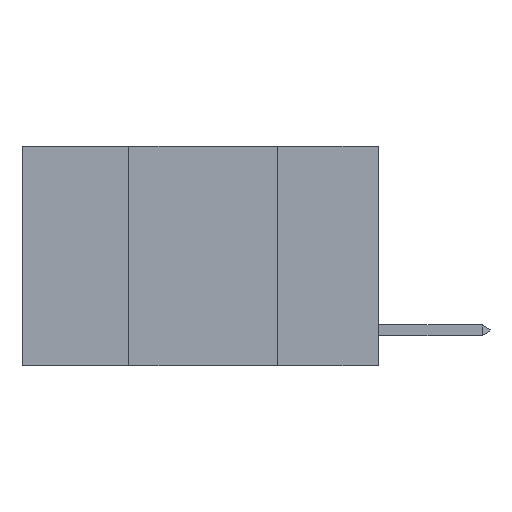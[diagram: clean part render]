
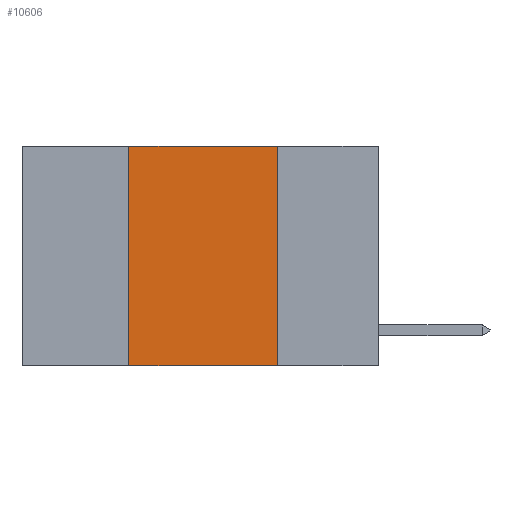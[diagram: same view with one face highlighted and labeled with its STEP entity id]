
A CAD part, left-side view. The second image highlights one B-rep face of the part: STEP entity #10606.
In plain terms, the highlighted planar face has unit normal (-1, 0, 0).
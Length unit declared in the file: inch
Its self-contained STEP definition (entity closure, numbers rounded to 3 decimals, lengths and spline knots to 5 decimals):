
#412 = VECTOR ( 'NONE', #18051, 39.37008 ) ;
#498 = DIRECTION ( 'NONE',  ( 0., -1., 0. ) ) ;
#578 = ORIENTED_EDGE ( 'NONE', *, *, #5093, .F. ) ;
#598 = DIRECTION ( 'NONE',  ( 0., 0., 1. ) ) ;
#825 = FACE_OUTER_BOUND ( 'NONE', #16294, .T. ) ;
#2417 = VERTEX_POINT ( 'NONE', #18025 ) ;
#2483 = DIRECTION ( 'NONE',  ( 0., 0., -1. ) ) ;
#4093 = VERTEX_POINT ( 'NONE', #6018 ) ;
#4453 = ORIENTED_EDGE ( 'NONE', *, *, #9075, .F. ) ;
#4703 = PLANE ( 'NONE',  #17337 ) ;
#5093 = EDGE_CURVE ( 'NONE', #11967, #4093, #12989, .T. ) ;
#6018 = CARTESIAN_POINT ( 'NONE',  ( 0., 0.17, 0. ) ) ;
#6133 = DIRECTION ( 'NONE',  ( 1., 0., 0. ) ) ;
#6457 = EDGE_CURVE ( 'NONE', #4093, #14872, #6820, .T. ) ;
#6820 = LINE ( 'NONE', #9618, #13377 ) ;
#6942 = CARTESIAN_POINT ( 'NONE',  ( 0., 0.6, -0.37 ) ) ;
#8101 = LINE ( 'NONE', #6942, #412 ) ;
#9075 = EDGE_CURVE ( 'NONE', #2417, #11967, #9873, .T. ) ;
#9618 = CARTESIAN_POINT ( 'NONE',  ( 0., 0.17, 0. ) ) ;
#9690 = CARTESIAN_POINT ( 'NONE',  ( 0., 0.42, 0. ) ) ;
#9694 = VECTOR ( 'NONE', #498, 39.37008 ) ;
#9873 = LINE ( 'NONE', #17492, #12734 ) ;
#10112 = CARTESIAN_POINT ( 'NONE',  ( 0., 0.17, -0.37 ) ) ;
#10606 = ADVANCED_FACE ( 'NONE', ( #825 ), #4703, .F. ) ;
#11967 = VERTEX_POINT ( 'NONE', #9690 ) ;
#11968 = ORIENTED_EDGE ( 'NONE', *, *, #16756, .T. ) ;
#12734 = VECTOR ( 'NONE', #598, 39.37008 ) ;
#12989 = LINE ( 'NONE', #17399, #9694 ) ;
#13377 = VECTOR ( 'NONE', #2483, 39.37008 ) ;
#14487 = CARTESIAN_POINT ( 'NONE',  ( 0., 0.6, 0. ) ) ;
#14872 = VERTEX_POINT ( 'NONE', #10112 ) ;
#15194 = ORIENTED_EDGE ( 'NONE', *, *, #6457, .F. ) ;
#15882 = DIRECTION ( 'NONE',  ( 0., 0., -1. ) ) ;
#16294 = EDGE_LOOP ( 'NONE', ( #15194, #578, #4453, #11968 ) ) ;
#16756 = EDGE_CURVE ( 'NONE', #2417, #14872, #8101, .T. ) ;
#17337 = AXIS2_PLACEMENT_3D ( 'NONE', #14487, #6133, #15882 ) ;
#17399 = CARTESIAN_POINT ( 'NONE',  ( 0., 0.6, 0. ) ) ;
#17492 = CARTESIAN_POINT ( 'NONE',  ( 0., 0.42, 0. ) ) ;
#18025 = CARTESIAN_POINT ( 'NONE',  ( 0., 0.42, -0.37 ) ) ;
#18051 = DIRECTION ( 'NONE',  ( 0., -1., 0. ) ) ;
